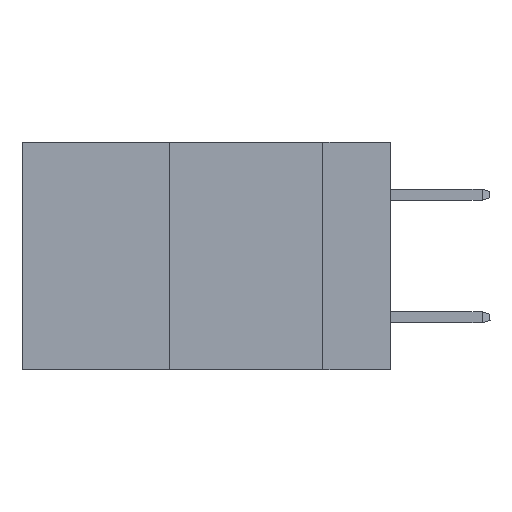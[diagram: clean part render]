
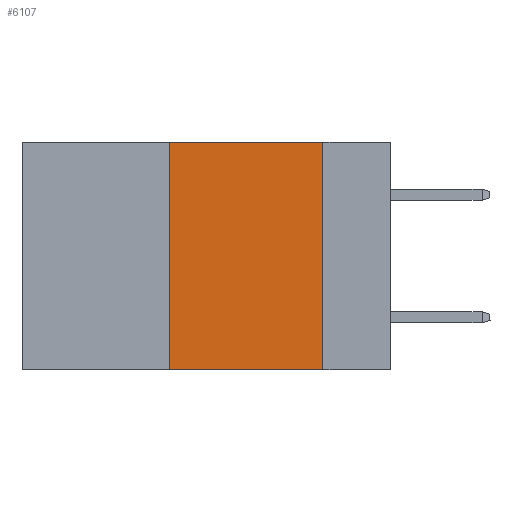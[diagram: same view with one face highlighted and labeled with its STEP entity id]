
A CAD part, left-side view. The second image highlights one B-rep face of the part: STEP entity #6107.
In plain terms, the highlighted planar face has unit normal (-1, 0, 0).
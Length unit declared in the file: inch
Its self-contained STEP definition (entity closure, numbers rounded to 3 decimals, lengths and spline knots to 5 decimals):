
#37 = FACE_OUTER_BOUND ( 'NONE', #3079, .T. ) ;
#554 = LINE ( 'NONE', #9451, #5129 ) ;
#820 = CARTESIAN_POINT ( 'NONE',  ( 0., 0.11, -0.37 ) ) ;
#1032 = CARTESIAN_POINT ( 'NONE',  ( 0., 0.36, 0. ) ) ;
#1619 = LINE ( 'NONE', #4594, #10340 ) ;
#1951 = DIRECTION ( 'NONE',  ( 0., 0., -1. ) ) ;
#2008 = CARTESIAN_POINT ( 'NONE',  ( 0., 0.36, -0.37 ) ) ;
#3064 = EDGE_CURVE ( 'NONE', #5132, #4819, #7845, .T. ) ;
#3079 = EDGE_LOOP ( 'NONE', ( #5687, #4038, #3758, #5152 ) ) ;
#3507 = LINE ( 'NONE', #5285, #9360 ) ;
#3532 = EDGE_CURVE ( 'NONE', #8361, #5508, #554, .T. ) ;
#3658 = EDGE_CURVE ( 'NONE', #5132, #5508, #1619, .T. ) ;
#3758 = ORIENTED_EDGE ( 'NONE', *, *, #3064, .F. ) ;
#4038 = ORIENTED_EDGE ( 'NONE', *, *, #9540, .F. ) ;
#4594 = CARTESIAN_POINT ( 'NONE',  ( 0., 0.6, -0.37 ) ) ;
#4819 = VERTEX_POINT ( 'NONE', #10170 ) ;
#5129 = VECTOR ( 'NONE', #1951, 39.37008 ) ;
#5132 = VERTEX_POINT ( 'NONE', #2008 ) ;
#5152 = ORIENTED_EDGE ( 'NONE', *, *, #3658, .T. ) ;
#5285 = CARTESIAN_POINT ( 'NONE',  ( 0., 0.6, 0. ) ) ;
#5417 = VECTOR ( 'NONE', #7818, 39.37008 ) ;
#5508 = VERTEX_POINT ( 'NONE', #820 ) ;
#5687 = ORIENTED_EDGE ( 'NONE', *, *, #3532, .F. ) ;
#6107 = ADVANCED_FACE ( 'NONE', ( #37 ), #9440, .F. ) ;
#6223 = AXIS2_PLACEMENT_3D ( 'NONE', #9430, #9420, #9399 ) ;
#7818 = DIRECTION ( 'NONE',  ( 0., 0., 1. ) ) ;
#7845 = LINE ( 'NONE', #1032, #5417 ) ;
#8361 = VERTEX_POINT ( 'NONE', #10918 ) ;
#9360 = VECTOR ( 'NONE', #10178, 39.37008 ) ;
#9399 = DIRECTION ( 'NONE',  ( 0., 0., -1. ) ) ;
#9420 = DIRECTION ( 'NONE',  ( 1., 0., 0. ) ) ;
#9426 = DIRECTION ( 'NONE',  ( 0., -1., 0. ) ) ;
#9430 = CARTESIAN_POINT ( 'NONE',  ( 0., 0.6, 0. ) ) ;
#9440 = PLANE ( 'NONE',  #6223 ) ;
#9451 = CARTESIAN_POINT ( 'NONE',  ( 0., 0.11, 0. ) ) ;
#9540 = EDGE_CURVE ( 'NONE', #4819, #8361, #3507, .T. ) ;
#10170 = CARTESIAN_POINT ( 'NONE',  ( 0., 0.36, 0. ) ) ;
#10178 = DIRECTION ( 'NONE',  ( 0., -1., 0. ) ) ;
#10340 = VECTOR ( 'NONE', #9426, 39.37008 ) ;
#10918 = CARTESIAN_POINT ( 'NONE',  ( 0., 0.11, 0. ) ) ;
